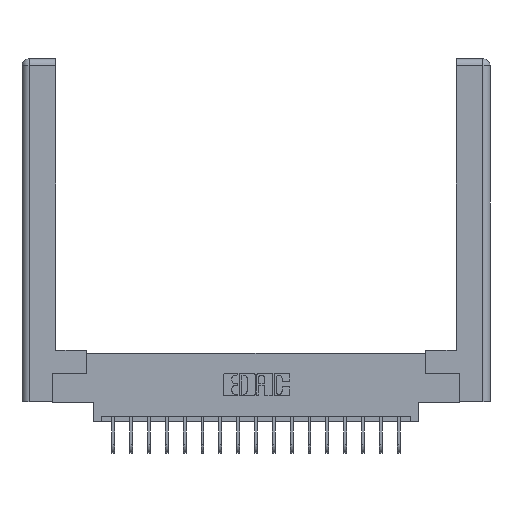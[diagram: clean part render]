
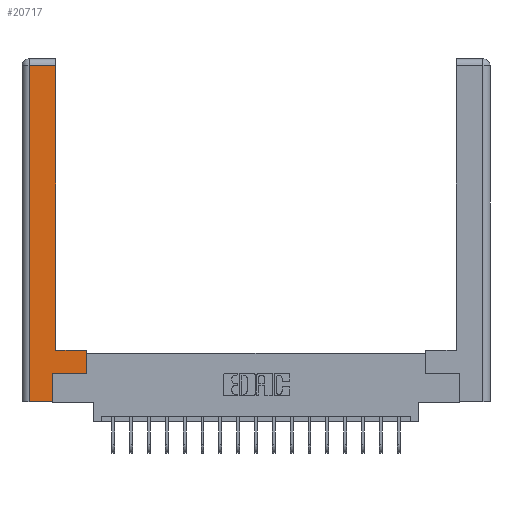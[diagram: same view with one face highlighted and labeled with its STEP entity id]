
A CAD part, top view. The second image highlights one B-rep face of the part: STEP entity #20717.
In plain terms, the highlighted planar face has unit normal (0, 0, 1).
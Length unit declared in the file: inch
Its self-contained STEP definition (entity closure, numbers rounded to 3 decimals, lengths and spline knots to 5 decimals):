
#329 = VERTEX_POINT ( 'NONE', #18668 ) ;
#544 = FACE_OUTER_BOUND ( 'NONE', #5253, .T. ) ;
#697 = ORIENTED_EDGE ( 'NONE', *, *, #15117, .T. ) ;
#876 = VECTOR ( 'NONE', #1447, 39.37008 ) ;
#1447 = DIRECTION ( 'NONE',  ( 0., 1., 0. ) ) ;
#1740 = LINE ( 'NONE', #18352, #11401 ) ;
#2897 = CARTESIAN_POINT ( 'NONE',  ( 0.0615, 2.94, 0. ) ) ;
#3395 = VECTOR ( 'NONE', #15982, 39.37008 ) ;
#3505 = ORIENTED_EDGE ( 'NONE', *, *, #17408, .T. ) ;
#3747 = CARTESIAN_POINT ( 'NONE',  ( 0.0615, 0., 0. ) ) ;
#4491 = LINE ( 'NONE', #3747, #19983 ) ;
#4508 = VECTOR ( 'NONE', #18811, 39.37008 ) ;
#4995 = EDGE_CURVE ( 'NONE', #11124, #13549, #15367, .T. ) ;
#5253 = EDGE_LOOP ( 'NONE', ( #17826, #20206, #3505, #5911, #19355, #15977, #697, #7876 ) ) ;
#5911 = ORIENTED_EDGE ( 'NONE', *, *, #4995, .T. ) ;
#6509 = PLANE ( 'NONE',  #10185 ) ;
#7027 = LINE ( 'NONE', #12801, #876 ) ;
#7491 = CARTESIAN_POINT ( 'NONE',  ( 0.565, 0.45, 0. ) ) ;
#7529 = CARTESIAN_POINT ( 'NONE',  ( 0.295, 0.45, 0. ) ) ;
#7830 = CARTESIAN_POINT ( 'NONE',  ( 0.265, 0., 0. ) ) ;
#7876 = ORIENTED_EDGE ( 'NONE', *, *, #17319, .T. ) ;
#8157 = DIRECTION ( 'NONE',  ( 0., 0., -1. ) ) ;
#8313 = CARTESIAN_POINT ( 'NONE',  ( 0., 0., 0. ) ) ;
#8597 = CARTESIAN_POINT ( 'NONE',  ( 0.0615, 0., 0. ) ) ;
#8849 = CARTESIAN_POINT ( 'NONE',  ( 0.265, 0., 0. ) ) ;
#8968 = VERTEX_POINT ( 'NONE', #8999 ) ;
#8999 = CARTESIAN_POINT ( 'NONE',  ( 0.565, 0.245, 0. ) ) ;
#10178 = DIRECTION ( 'NONE',  ( 0., -1., 0. ) ) ;
#10185 = AXIS2_PLACEMENT_3D ( 'NONE', #8313, #8157, #19522 ) ;
#10487 = LINE ( 'NONE', #2897, #18083 ) ;
#10566 = DIRECTION ( 'NONE',  ( 0., 1., 0. ) ) ;
#10934 = CARTESIAN_POINT ( 'NONE',  ( 0.295, 0.45, 0. ) ) ;
#11124 = VERTEX_POINT ( 'NONE', #8597 ) ;
#11401 = VECTOR ( 'NONE', #13438, 39.37008 ) ;
#11729 = EDGE_CURVE ( 'NONE', #12457, #329, #1740, .T. ) ;
#11795 = VECTOR ( 'NONE', #17328, 39.37008 ) ;
#12439 = DIRECTION ( 'NONE',  ( -1., 0., 0. ) ) ;
#12457 = VERTEX_POINT ( 'NONE', #10934 ) ;
#12801 = CARTESIAN_POINT ( 'NONE',  ( 0.265, 0.245, 0. ) ) ;
#12929 = VERTEX_POINT ( 'NONE', #7491 ) ;
#13438 = DIRECTION ( 'NONE',  ( 0., 1., 0. ) ) ;
#13549 = VERTEX_POINT ( 'NONE', #7830 ) ;
#13746 = CARTESIAN_POINT ( 'NONE',  ( 0.565, 0.45, 0. ) ) ;
#15062 = CARTESIAN_POINT ( 'NONE',  ( 0.565, 0.245, 0. ) ) ;
#15117 = EDGE_CURVE ( 'NONE', #8968, #12929, #20636, .T. ) ;
#15218 = CARTESIAN_POINT ( 'NONE',  ( 0.265, 0.245, 0. ) ) ;
#15367 = LINE ( 'NONE', #8849, #11795 ) ;
#15854 = EDGE_CURVE ( 'NONE', #329, #17345, #10487, .T. ) ;
#15977 = ORIENTED_EDGE ( 'NONE', *, *, #19230, .T. ) ;
#15982 = DIRECTION ( 'NONE',  ( 1., 0., 0. ) ) ;
#17319 = EDGE_CURVE ( 'NONE', #12929, #12457, #20735, .T. ) ;
#17328 = DIRECTION ( 'NONE',  ( 1., 0., 0. ) ) ;
#17345 = VERTEX_POINT ( 'NONE', #18956 ) ;
#17408 = EDGE_CURVE ( 'NONE', #17345, #11124, #4491, .T. ) ;
#17826 = ORIENTED_EDGE ( 'NONE', *, *, #11729, .T. ) ;
#18083 = VECTOR ( 'NONE', #12439, 39.37008 ) ;
#18352 = CARTESIAN_POINT ( 'NONE',  ( 0.295, 3., 0. ) ) ;
#18356 = EDGE_CURVE ( 'NONE', #13549, #20340, #7027, .T. ) ;
#18369 = VECTOR ( 'NONE', #10566, 39.37008 ) ;
#18668 = CARTESIAN_POINT ( 'NONE',  ( 0.295, 2.94, 0. ) ) ;
#18811 = DIRECTION ( 'NONE',  ( -1., 0., 0. ) ) ;
#18956 = CARTESIAN_POINT ( 'NONE',  ( 0.0615, 2.94, 0. ) ) ;
#19230 = EDGE_CURVE ( 'NONE', #20340, #8968, #19408, .T. ) ;
#19355 = ORIENTED_EDGE ( 'NONE', *, *, #18356, .T. ) ;
#19408 = LINE ( 'NONE', #15062, #3395 ) ;
#19522 = DIRECTION ( 'NONE',  ( -1., 0., 0. ) ) ;
#19983 = VECTOR ( 'NONE', #10178, 39.37008 ) ;
#20206 = ORIENTED_EDGE ( 'NONE', *, *, #15854, .T. ) ;
#20340 = VERTEX_POINT ( 'NONE', #15218 ) ;
#20636 = LINE ( 'NONE', #13746, #18369 ) ;
#20717 = ADVANCED_FACE ( 'NONE', ( #544 ), #6509, .F. ) ;
#20735 = LINE ( 'NONE', #7529, #4508 ) ;
